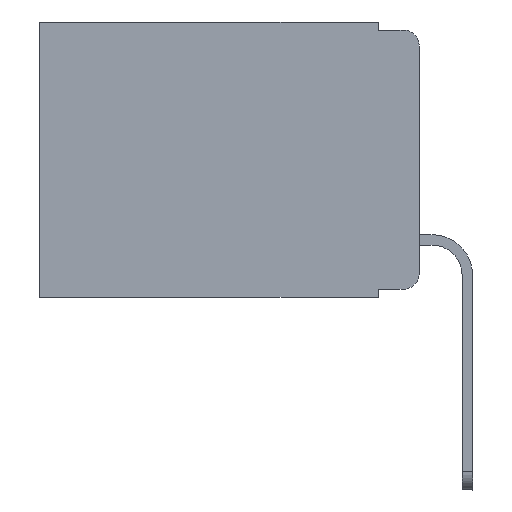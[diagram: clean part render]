
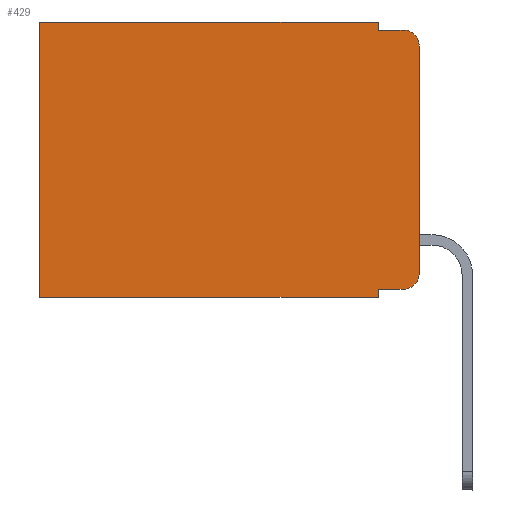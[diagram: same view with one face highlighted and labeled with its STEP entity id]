
A CAD part, left-side view. The second image highlights one B-rep face of the part: STEP entity #429.
In plain terms, the highlighted planar face has unit normal (-1, 0, 0).
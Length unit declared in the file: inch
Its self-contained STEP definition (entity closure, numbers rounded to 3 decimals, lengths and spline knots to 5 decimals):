
#233 = ORIENTED_EDGE ( 'NONE', *, *, #3135, .F. ) ;
#379 = ORIENTED_EDGE ( 'NONE', *, *, #7718, .T. ) ;
#429 = ADVANCED_FACE ( 'NONE', ( #3217 ), #6788, .F. ) ;
#469 = LINE ( 'NONE', #1412, #9073 ) ;
#595 = CARTESIAN_POINT ( 'NONE',  ( 0.298, 0.051, -0.333 ) ) ;
#1224 = VECTOR ( 'NONE', #10644, 39.37008 ) ;
#1412 = CARTESIAN_POINT ( 'NONE',  ( 0.298, 0.051, -0.333 ) ) ;
#1461 = EDGE_CURVE ( 'NONE', #9556, #9087, #3412, .T. ) ;
#1476 = DIRECTION ( 'NONE',  ( 0., 0., -1. ) ) ;
#1585 = DIRECTION ( 'NONE',  ( -1., 0., 0. ) ) ;
#2026 = EDGE_LOOP ( 'NONE', ( #9402, #5736, #5346, #233, #9462, #379, #8114, #3115, #4695, #10884 ) ) ;
#2467 = CARTESIAN_POINT ( 'NONE',  ( 0.298, 0.051, 0. ) ) ;
#2744 = VERTEX_POINT ( 'NONE', #6167 ) ;
#2791 = VECTOR ( 'NONE', #7335, 39.37008 ) ;
#2796 = VERTEX_POINT ( 'NONE', #6455 ) ;
#2836 = CARTESIAN_POINT ( 'NONE',  ( 0.298, 0.02, -0.313 ) ) ;
#2986 = EDGE_CURVE ( 'NONE', #9556, #7205, #469, .T. ) ;
#3115 = ORIENTED_EDGE ( 'NONE', *, *, #1461, .F. ) ;
#3133 = VECTOR ( 'NONE', #5184, 39.37008 ) ;
#3135 = EDGE_CURVE ( 'NONE', #2796, #10499, #7910, .T. ) ;
#3154 = EDGE_CURVE ( 'NONE', #7609, #9914, #6080, .T. ) ;
#3217 = FACE_OUTER_BOUND ( 'NONE', #2026, .T. ) ;
#3412 = LINE ( 'NONE', #3524, #9997 ) ;
#3447 = CARTESIAN_POINT ( 'NONE',  ( 0.298, 0.051, -0.01 ) ) ;
#3464 = CIRCLE ( 'NONE', #4011, 0.02 ) ;
#3524 = CARTESIAN_POINT ( 'NONE',  ( 0.298, 0.051, 0. ) ) ;
#3571 = AXIS2_PLACEMENT_3D ( 'NONE', #8589, #6842, #8410 ) ;
#3598 = LINE ( 'NONE', #7990, #4992 ) ;
#3696 = CARTESIAN_POINT ( 'NONE',  ( 0.298, 0.473, 0. ) ) ;
#3896 = DIRECTION ( 'NONE',  ( -1., 0., 0. ) ) ;
#4011 = AXIS2_PLACEMENT_3D ( 'NONE', #2836, #3896, #8158 ) ;
#4214 = EDGE_CURVE ( 'NONE', #7205, #2744, #3464, .T. ) ;
#4326 = EDGE_CURVE ( 'NONE', #9087, #7518, #9355, .T. ) ;
#4695 = ORIENTED_EDGE ( 'NONE', *, *, #2986, .T. ) ;
#4700 = VECTOR ( 'NONE', #7765, 39.37008 ) ;
#4992 = VECTOR ( 'NONE', #6353, 39.37008 ) ;
#5145 = CARTESIAN_POINT ( 'NONE',  ( 0.298, 0.02, -0.01 ) ) ;
#5184 = DIRECTION ( 'NONE',  ( 0., 0., -1. ) ) ;
#5346 = ORIENTED_EDGE ( 'NONE', *, *, #7587, .F. ) ;
#5525 = AXIS2_PLACEMENT_3D ( 'NONE', #6027, #1585, #1476 ) ;
#5699 = LINE ( 'NONE', #9097, #2791 ) ;
#5736 = ORIENTED_EDGE ( 'NONE', *, *, #3154, .T. ) ;
#6013 = EDGE_CURVE ( 'NONE', #2796, #11076, #5699, .T. ) ;
#6027 = CARTESIAN_POINT ( 'NONE',  ( 0.298, 0.02, -0.03 ) ) ;
#6080 = CIRCLE ( 'NONE', #5525, 0.02 ) ;
#6167 = CARTESIAN_POINT ( 'NONE',  ( 0.298, 0., -0.313 ) ) ;
#6353 = DIRECTION ( 'NONE',  ( 0., -1., 0. ) ) ;
#6455 = CARTESIAN_POINT ( 'NONE',  ( 0.298, 0.051, 0. ) ) ;
#6534 = CARTESIAN_POINT ( 'NONE',  ( 0.298, 0.473, 0. ) ) ;
#6740 = LINE ( 'NONE', #11104, #3133 ) ;
#6788 = PLANE ( 'NONE',  #3571 ) ;
#6842 = DIRECTION ( 'NONE',  ( 1., 0., 0. ) ) ;
#7205 = VERTEX_POINT ( 'NONE', #10642 ) ;
#7335 = DIRECTION ( 'NONE',  ( 0., 1., 0. ) ) ;
#7380 = EDGE_CURVE ( 'NONE', #7609, #2744, #6740, .T. ) ;
#7409 = LINE ( 'NONE', #6534, #7813 ) ;
#7518 = VERTEX_POINT ( 'NONE', #8874 ) ;
#7587 = EDGE_CURVE ( 'NONE', #10499, #9914, #3598, .T. ) ;
#7609 = VERTEX_POINT ( 'NONE', #9830 ) ;
#7718 = EDGE_CURVE ( 'NONE', #11076, #7518, #7409, .T. ) ;
#7765 = DIRECTION ( 'NONE',  ( 0., 1., 0. ) ) ;
#7813 = VECTOR ( 'NONE', #8442, 39.37008 ) ;
#7910 = LINE ( 'NONE', #2467, #1224 ) ;
#7990 = CARTESIAN_POINT ( 'NONE',  ( 0.298, 0.051, -0.01 ) ) ;
#8114 = ORIENTED_EDGE ( 'NONE', *, *, #4326, .F. ) ;
#8158 = DIRECTION ( 'NONE',  ( 0., 0., -1. ) ) ;
#8410 = DIRECTION ( 'NONE',  ( 0., 0., -1. ) ) ;
#8442 = DIRECTION ( 'NONE',  ( 0., 0., -1. ) ) ;
#8504 = CARTESIAN_POINT ( 'NONE',  ( 0.298, 0., -0.343 ) ) ;
#8589 = CARTESIAN_POINT ( 'NONE',  ( 0.298, 0., 0. ) ) ;
#8874 = CARTESIAN_POINT ( 'NONE',  ( 0.298, 0.473, -0.343 ) ) ;
#9073 = VECTOR ( 'NONE', #11246, 39.37008 ) ;
#9087 = VERTEX_POINT ( 'NONE', #9427 ) ;
#9097 = CARTESIAN_POINT ( 'NONE',  ( 0.298, 0., 0. ) ) ;
#9355 = LINE ( 'NONE', #8504, #4700 ) ;
#9402 = ORIENTED_EDGE ( 'NONE', *, *, #7380, .F. ) ;
#9427 = CARTESIAN_POINT ( 'NONE',  ( 0.298, 0.051, -0.343 ) ) ;
#9462 = ORIENTED_EDGE ( 'NONE', *, *, #6013, .T. ) ;
#9556 = VERTEX_POINT ( 'NONE', #595 ) ;
#9793 = DIRECTION ( 'NONE',  ( 0., 0., -1. ) ) ;
#9830 = CARTESIAN_POINT ( 'NONE',  ( 0.298, 0., -0.03 ) ) ;
#9914 = VERTEX_POINT ( 'NONE', #5145 ) ;
#9997 = VECTOR ( 'NONE', #9793, 39.37008 ) ;
#10499 = VERTEX_POINT ( 'NONE', #3447 ) ;
#10642 = CARTESIAN_POINT ( 'NONE',  ( 0.298, 0.02, -0.333 ) ) ;
#10644 = DIRECTION ( 'NONE',  ( 0., 0., -1. ) ) ;
#10884 = ORIENTED_EDGE ( 'NONE', *, *, #4214, .T. ) ;
#11076 = VERTEX_POINT ( 'NONE', #3696 ) ;
#11104 = CARTESIAN_POINT ( 'NONE',  ( 0.298, 0., 0. ) ) ;
#11246 = DIRECTION ( 'NONE',  ( 0., -1., 0. ) ) ;
